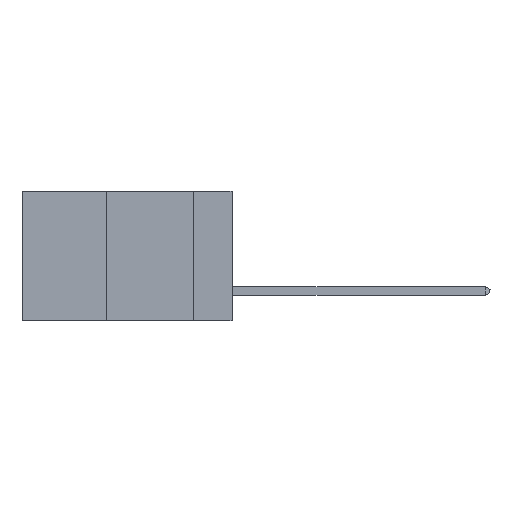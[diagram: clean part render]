
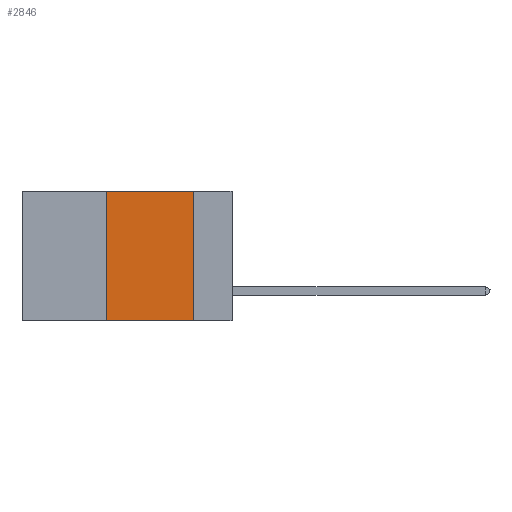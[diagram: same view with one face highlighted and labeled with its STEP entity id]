
A CAD part, left-side view. The second image highlights one B-rep face of the part: STEP entity #2846.
In plain terms, the highlighted planar face has unit normal (-1, 0, 0).
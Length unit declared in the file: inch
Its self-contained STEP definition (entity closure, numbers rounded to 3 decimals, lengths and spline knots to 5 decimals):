
#200 = VERTEX_POINT ( 'NONE', #4384 ) ;
#2683 = PLANE ( 'NONE',  #32162 ) ;
#2846 = ADVANCED_FACE ( 'NONE', ( #23620 ), #2683, .F. ) ;
#3032 = DIRECTION ( 'NONE',  ( 0., 0., -1. ) ) ;
#4384 = CARTESIAN_POINT ( 'NONE',  ( 0., 0.11, 0. ) ) ;
#5156 = LINE ( 'NONE', #5904, #38137 ) ;
#5683 = VECTOR ( 'NONE', #19908, 39.37008 ) ;
#5904 = CARTESIAN_POINT ( 'NONE',  ( 0., 0.11, 0. ) ) ;
#5942 = DIRECTION ( 'NONE',  ( 1., 0., 0. ) ) ;
#5995 = EDGE_CURVE ( 'NONE', #6731, #26717, #31237, .T. ) ;
#6731 = VERTEX_POINT ( 'NONE', #30295 ) ;
#7826 = CARTESIAN_POINT ( 'NONE',  ( 0., 0.6, -0.37 ) ) ;
#9303 = LINE ( 'NONE', #30732, #26970 ) ;
#10767 = DIRECTION ( 'NONE',  ( 0., -1., 0. ) ) ;
#13885 = ORIENTED_EDGE ( 'NONE', *, *, #23127, .F. ) ;
#14755 = DIRECTION ( 'NONE',  ( 0., 0., -1. ) ) ;
#15818 = LINE ( 'NONE', #22904, #5683 ) ;
#15856 = CARTESIAN_POINT ( 'NONE',  ( 0., 0.11, -0.37 ) ) ;
#17720 = CARTESIAN_POINT ( 'NONE',  ( 0., 0.6, 0. ) ) ;
#17911 = ORIENTED_EDGE ( 'NONE', *, *, #5995, .T. ) ;
#18507 = VERTEX_POINT ( 'NONE', #38532 ) ;
#19908 = DIRECTION ( 'NONE',  ( 0., -1., 0. ) ) ;
#20716 = ORIENTED_EDGE ( 'NONE', *, *, #27678, .F. ) ;
#22161 = EDGE_LOOP ( 'NONE', ( #13885, #20716, #29588, #17911 ) ) ;
#22904 = CARTESIAN_POINT ( 'NONE',  ( 0., 0.6, 0. ) ) ;
#23127 = EDGE_CURVE ( 'NONE', #200, #26717, #5156, .T. ) ;
#23398 = VECTOR ( 'NONE', #10767, 39.37008 ) ;
#23620 = FACE_OUTER_BOUND ( 'NONE', #22161, .T. ) ;
#26717 = VERTEX_POINT ( 'NONE', #15856 ) ;
#26970 = VECTOR ( 'NONE', #36908, 39.37008 ) ;
#27678 = EDGE_CURVE ( 'NONE', #18507, #200, #15818, .T. ) ;
#27973 = EDGE_CURVE ( 'NONE', #6731, #18507, #9303, .T. ) ;
#29588 = ORIENTED_EDGE ( 'NONE', *, *, #27973, .F. ) ;
#30295 = CARTESIAN_POINT ( 'NONE',  ( 0., 0.36, -0.37 ) ) ;
#30732 = CARTESIAN_POINT ( 'NONE',  ( 0., 0.36, 0. ) ) ;
#31237 = LINE ( 'NONE', #7826, #23398 ) ;
#32162 = AXIS2_PLACEMENT_3D ( 'NONE', #17720, #5942, #3032 ) ;
#36908 = DIRECTION ( 'NONE',  ( 0., 0., 1. ) ) ;
#38137 = VECTOR ( 'NONE', #14755, 39.37008 ) ;
#38532 = CARTESIAN_POINT ( 'NONE',  ( 0., 0.36, 0. ) ) ;
